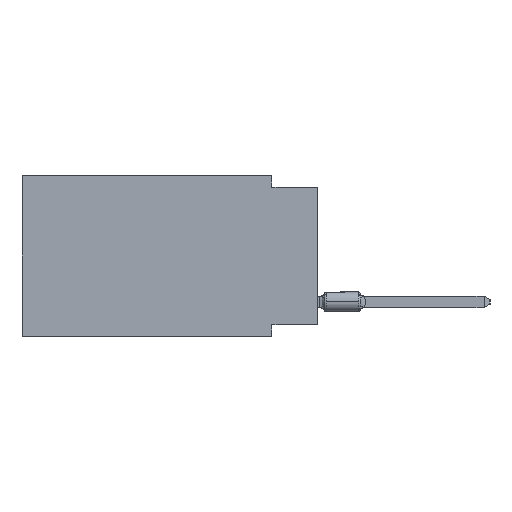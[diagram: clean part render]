
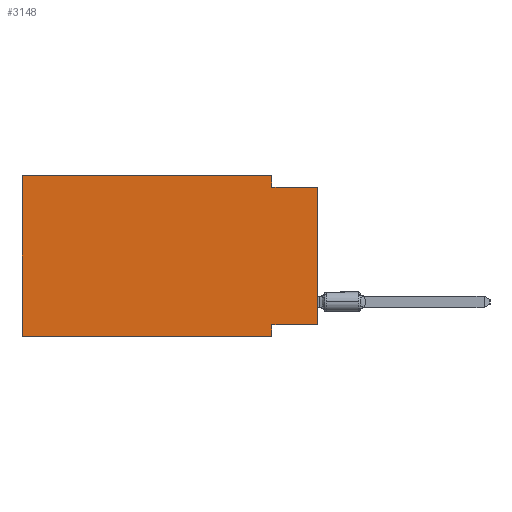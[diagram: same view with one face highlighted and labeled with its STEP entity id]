
A CAD part, left-side view. The second image highlights one B-rep face of the part: STEP entity #3148.
In plain terms, the highlighted planar face has unit normal (-1, 0, 0).
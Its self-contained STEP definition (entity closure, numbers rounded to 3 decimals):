
#523 = VECTOR ( 'NONE', #48794, 1000. ) ;
#726 = LINE ( 'NONE', #10447, #56785 ) ;
#1169 = VECTOR ( 'NONE', #47347, 1000. ) ;
#2443 = EDGE_CURVE ( 'NONE', #27982, #25717, #58921, .T. ) ;
#2447 = VERTEX_POINT ( 'NONE', #57933 ) ;
#3148 = ADVANCED_FACE ( 'NONE', ( #59143 ), #13740, .F. ) ;
#3794 = AXIS2_PLACEMENT_3D ( 'NONE', #9031, #14703, #24427 ) ;
#3843 = ORIENTED_EDGE ( 'NONE', *, *, #51427, .F. ) ;
#5116 = EDGE_CURVE ( 'NONE', #8542, #63319, #36946, .T. ) ;
#5987 = VECTOR ( 'NONE', #46972, 1000. ) ;
#6362 = CARTESIAN_POINT ( 'NONE',  ( 0., 0., -8.255 ) ) ;
#6782 = CARTESIAN_POINT ( 'NONE',  ( 0., 2.54, -0.635 ) ) ;
#8157 = DIRECTION ( 'NONE',  ( 0., 1., 0. ) ) ;
#8542 = VERTEX_POINT ( 'NONE', #24580 ) ;
#8816 = CARTESIAN_POINT ( 'NONE',  ( 0., 0., -0.635 ) ) ;
#8925 = CARTESIAN_POINT ( 'NONE',  ( 0., 2.54, 0. ) ) ;
#9031 = CARTESIAN_POINT ( 'NONE',  ( 0., 16.383, 0. ) ) ;
#9426 = EDGE_CURVE ( 'NONE', #57929, #28787, #16622, .T. ) ;
#10248 = ORIENTED_EDGE ( 'NONE', *, *, #43012, .T. ) ;
#10447 = CARTESIAN_POINT ( 'NONE',  ( 0., 0., 0. ) ) ;
#13740 = PLANE ( 'NONE',  #3794 ) ;
#14703 = DIRECTION ( 'NONE',  ( 1., 0., 0. ) ) ;
#15685 = ORIENTED_EDGE ( 'NONE', *, *, #52101, .T. ) ;
#16317 = EDGE_CURVE ( 'NONE', #28787, #42957, #39474, .T. ) ;
#16622 = LINE ( 'NONE', #37309, #1169 ) ;
#18140 = DIRECTION ( 'NONE',  ( 0., -1., 0. ) ) ;
#20937 = DIRECTION ( 'NONE',  ( 0., 0., 1. ) ) ;
#22267 = LINE ( 'NONE', #22602, #5987 ) ;
#22602 = CARTESIAN_POINT ( 'NONE',  ( 0., 16.383, -8.89 ) ) ;
#23480 = CARTESIAN_POINT ( 'NONE',  ( 0., 0., -0.635 ) ) ;
#23737 = LINE ( 'NONE', #33423, #523 ) ;
#24427 = DIRECTION ( 'NONE',  ( 0., 0., -1. ) ) ;
#24580 = CARTESIAN_POINT ( 'NONE',  ( 0., 16.383, -8.89 ) ) ;
#25717 = VERTEX_POINT ( 'NONE', #32261 ) ;
#25944 = CARTESIAN_POINT ( 'NONE',  ( 0., 16.383, 0. ) ) ;
#27982 = VERTEX_POINT ( 'NONE', #6362 ) ;
#28787 = VERTEX_POINT ( 'NONE', #6782 ) ;
#30574 = ORIENTED_EDGE ( 'NONE', *, *, #5116, .F. ) ;
#30842 = DIRECTION ( 'NONE',  ( 0., 0., 1. ) ) ;
#32261 = CARTESIAN_POINT ( 'NONE',  ( 0., 2.54, -8.255 ) ) ;
#32588 = VECTOR ( 'NONE', #8157, 1000. ) ;
#33423 = CARTESIAN_POINT ( 'NONE',  ( 0., 16.383, 0. ) ) ;
#33887 = CARTESIAN_POINT ( 'NONE',  ( 0., 0., -8.255 ) ) ;
#36946 = LINE ( 'NONE', #25944, #56370 ) ;
#36997 = ORIENTED_EDGE ( 'NONE', *, *, #16317, .F. ) ;
#37309 = CARTESIAN_POINT ( 'NONE',  ( 0., 2.54, 0. ) ) ;
#39474 = LINE ( 'NONE', #23480, #64273 ) ;
#40254 = EDGE_CURVE ( 'NONE', #25717, #2447, #62690, .T. ) ;
#42957 = VERTEX_POINT ( 'NONE', #8816 ) ;
#43012 = EDGE_CURVE ( 'NONE', #27982, #42957, #726, .T. ) ;
#46138 = ORIENTED_EDGE ( 'NONE', *, *, #2443, .F. ) ;
#46577 = EDGE_LOOP ( 'NONE', ( #10248, #36997, #56264, #3843, #30574, #15685, #52127, #46138 ) ) ;
#46972 = DIRECTION ( 'NONE',  ( 0., -1., 0. ) ) ;
#47347 = DIRECTION ( 'NONE',  ( 0., 0., -1. ) ) ;
#48537 = CARTESIAN_POINT ( 'NONE',  ( 0., 16.383, 0. ) ) ;
#48794 = DIRECTION ( 'NONE',  ( 0., -1., 0. ) ) ;
#51427 = EDGE_CURVE ( 'NONE', #63319, #57929, #23737, .T. ) ;
#52101 = EDGE_CURVE ( 'NONE', #8542, #2447, #22267, .T. ) ;
#52127 = ORIENTED_EDGE ( 'NONE', *, *, #40254, .F. ) ;
#56264 = ORIENTED_EDGE ( 'NONE', *, *, #9426, .F. ) ;
#56370 = VECTOR ( 'NONE', #20937, 1000. ) ;
#56785 = VECTOR ( 'NONE', #30842, 1000. ) ;
#57675 = DIRECTION ( 'NONE',  ( 0., 0., -1. ) ) ;
#57929 = VERTEX_POINT ( 'NONE', #8925 ) ;
#57933 = CARTESIAN_POINT ( 'NONE',  ( 0., 2.54, -8.89 ) ) ;
#58921 = LINE ( 'NONE', #33887, #32588 ) ;
#59143 = FACE_OUTER_BOUND ( 'NONE', #46577, .T. ) ;
#62690 = LINE ( 'NONE', #63020, #63887 ) ;
#63020 = CARTESIAN_POINT ( 'NONE',  ( 0., 2.54, -8.89 ) ) ;
#63319 = VERTEX_POINT ( 'NONE', #48537 ) ;
#63887 = VECTOR ( 'NONE', #57675, 1000. ) ;
#64273 = VECTOR ( 'NONE', #18140, 1000. ) ;
